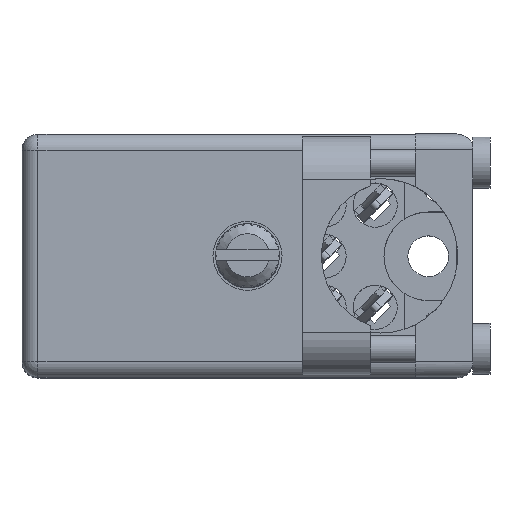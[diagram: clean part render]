
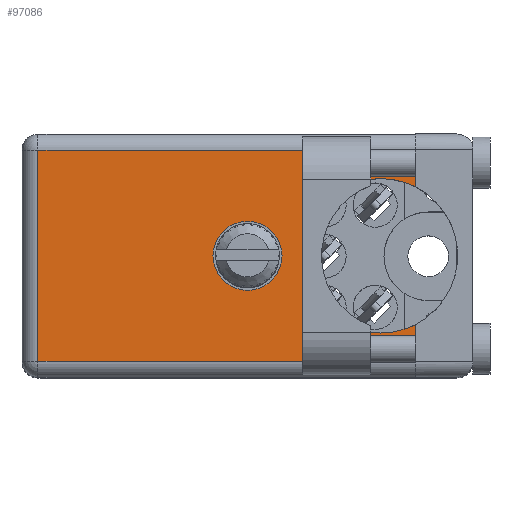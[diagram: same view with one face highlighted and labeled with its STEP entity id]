
A CAD part, top view. The second image highlights one B-rep face of the part: STEP entity #97086.
In plain terms, the highlighted face is planar.
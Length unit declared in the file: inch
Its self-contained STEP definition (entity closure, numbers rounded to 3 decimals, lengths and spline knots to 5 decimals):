
#646 = EDGE_CURVE ( 'NONE', #20752, #139106, #7418, .T. ) ;
#1485 = CARTESIAN_POINT ( 'NONE',  ( 0.6625, 0.906, -0.256 ) ) ;
#4443 = DIRECTION ( 'NONE',  ( 1., 0., 0. ) ) ;
#6586 = EDGE_CURVE ( 'NONE', #76998, #175186, #181791, .T. ) ;
#7418 = CIRCLE ( 'NONE', #58243, 0.227 ) ;
#10437 = CARTESIAN_POINT ( 'NONE',  ( 1.155, 0.906, 0. ) ) ;
#11727 = AXIS2_PLACEMENT_3D ( 'NONE', #88166, #17002, #131221 ) ;
#14114 = CARTESIAN_POINT ( 'NONE',  ( 1.155, 0.906, -0.047 ) ) ;
#14472 = FACE_OUTER_BOUND ( 'NONE', #15183, .T. ) ;
#15183 = EDGE_LOOP ( 'NONE', ( #36356, #139949, #70295, #163960, #52545, #22296, #155546, #24495 ) ) ;
#16550 = CARTESIAN_POINT ( 'NONE',  ( 1.053, 0.906, -0.1305 ) ) ;
#17002 = DIRECTION ( 'NONE',  ( 0., 1., 0. ) ) ;
#20700 = DIRECTION ( 'NONE',  ( 0., 0., 1. ) ) ;
#20752 = VERTEX_POINT ( 'NONE', #16550 ) ;
#22296 = ORIENTED_EDGE ( 'NONE', *, *, #646, .F. ) ;
#24495 = ORIENTED_EDGE ( 'NONE', *, *, #178279, .F. ) ;
#24763 = CIRCLE ( 'NONE', #78447, 0.227 ) ;
#27270 = LINE ( 'NONE', #14114, #47013 ) ;
#29269 = DIRECTION ( 'NONE',  ( 0., 1., 0. ) ) ;
#30152 = CARTESIAN_POINT ( 'NONE',  ( 1.155, 0.906, -0.047 ) ) ;
#33833 = DIRECTION ( 'NONE',  ( 0., 1., 0. ) ) ;
#36356 = ORIENTED_EDGE ( 'NONE', *, *, #183359, .F. ) ;
#37097 = CARTESIAN_POINT ( 'NONE',  ( 0.047, 0.906, -0.668 ) ) ;
#41361 = CARTESIAN_POINT ( 'NONE',  ( 1.053, 0.906, -0.3575 ) ) ;
#44445 = DIRECTION ( 'NONE',  ( 0., 1., 0. ) ) ;
#47013 = VECTOR ( 'NONE', #4443, 39.37008 ) ;
#47773 = VECTOR ( 'NONE', #182708, 39.37008 ) ;
#49642 = CARTESIAN_POINT ( 'NONE',  ( 1.053, 0.906, -0.3575 ) ) ;
#50746 = EDGE_CURVE ( 'NONE', #139106, #70561, #105013, .T. ) ;
#52545 = ORIENTED_EDGE ( 'NONE', *, *, #50746, .F. ) ;
#56371 = CARTESIAN_POINT ( 'NONE',  ( 1.155, 0.906, -0.56029 ) ) ;
#58243 = AXIS2_PLACEMENT_3D ( 'NONE', #49642, #178923, #106756 ) ;
#59424 = VERTEX_POINT ( 'NONE', #1485 ) ;
#65702 = DIRECTION ( 'NONE',  ( 0., 0., 1. ) ) ;
#70295 = ORIENTED_EDGE ( 'NONE', *, *, #6586, .T. ) ;
#70561 = VERTEX_POINT ( 'NONE', #30152 ) ;
#74352 = PLANE ( 'NONE',  #159305 ) ;
#75418 = CARTESIAN_POINT ( 'NONE',  ( 0.047, 0.906, -0.047 ) ) ;
#76998 = VERTEX_POINT ( 'NONE', #37097 ) ;
#77812 = CARTESIAN_POINT ( 'NONE',  ( 0.6625, 0.906, -0.3575 ) ) ;
#78376 = EDGE_CURVE ( 'NONE', #175186, #70561, #27270, .T. ) ;
#78447 = AXIS2_PLACEMENT_3D ( 'NONE', #101325, #29269, #103158 ) ;
#85336 = DIRECTION ( 'NONE',  ( 0., 1., 0. ) ) ;
#87816 = ORIENTED_EDGE ( 'NONE', *, *, #140770, .F. ) ;
#88141 = CIRCLE ( 'NONE', #163008, 0.1015 ) ;
#88166 = CARTESIAN_POINT ( 'NONE',  ( 0.6625, 0.906, -0.3575 ) ) ;
#97086 = ADVANCED_FACE ( 'NONE', ( #14472, #114687 ), #74352, .T. ) ;
#101325 = CARTESIAN_POINT ( 'NONE',  ( 1.053, 0.906, -0.3575 ) ) ;
#102247 = ORIENTED_EDGE ( 'NONE', *, *, #109840, .F. ) ;
#103146 = EDGE_LOOP ( 'NONE', ( #87816, #102247 ) ) ;
#103158 = DIRECTION ( 'NONE',  ( 0., 0., 1. ) ) ;
#105013 = LINE ( 'NONE', #175330, #146068 ) ;
#106756 = DIRECTION ( 'NONE',  ( 0., 0., 1. ) ) ;
#109840 = EDGE_CURVE ( 'NONE', #144207, #59424, #88141, .T. ) ;
#114687 = FACE_BOUND ( 'NONE', #103146, .T. ) ;
#115420 = EDGE_CURVE ( 'NONE', #122422, #76998, #164955, .T. ) ;
#116433 = AXIS2_PLACEMENT_3D ( 'NONE', #41361, #85336, #139667 ) ;
#119280 = VERTEX_POINT ( 'NONE', #56371 ) ;
#122422 = VERTEX_POINT ( 'NONE', #173773 ) ;
#125509 = CARTESIAN_POINT ( 'NONE',  ( 0.047, 0.906, -0.715 ) ) ;
#126523 = LINE ( 'NONE', #10437, #159487 ) ;
#128112 = CARTESIAN_POINT ( 'NONE',  ( 1.053, 0.906, -0.5845 ) ) ;
#129645 = DIRECTION ( 'NONE',  ( 0., 0., 1. ) ) ;
#131221 = DIRECTION ( 'NONE',  ( 0., 0., 1. ) ) ;
#132829 = EDGE_CURVE ( 'NONE', #179733, #20752, #140189, .T. ) ;
#132940 = CARTESIAN_POINT ( 'NONE',  ( 0.6625, 0.906, -0.459 ) ) ;
#134314 = CIRCLE ( 'NONE', #11727, 0.1015 ) ;
#139106 = VERTEX_POINT ( 'NONE', #155406 ) ;
#139667 = DIRECTION ( 'NONE',  ( 0., 0., 1. ) ) ;
#139949 = ORIENTED_EDGE ( 'NONE', *, *, #115420, .T. ) ;
#140189 = CIRCLE ( 'NONE', #116433, 0.227 ) ;
#140770 = EDGE_CURVE ( 'NONE', #59424, #144207, #134314, .T. ) ;
#144207 = VERTEX_POINT ( 'NONE', #132940 ) ;
#146068 = VECTOR ( 'NONE', #146231, 39.37008 ) ;
#146231 = DIRECTION ( 'NONE',  ( 0., 0., 1. ) ) ;
#149011 = DIRECTION ( 'NONE',  ( -1., 0., 0. ) ) ;
#155406 = CARTESIAN_POINT ( 'NONE',  ( 1.155, 0.906, -0.15471 ) ) ;
#155546 = ORIENTED_EDGE ( 'NONE', *, *, #132829, .F. ) ;
#158686 = CARTESIAN_POINT ( 'NONE',  ( 0., 0.906, -0.715 ) ) ;
#159305 = AXIS2_PLACEMENT_3D ( 'NONE', #158686, #44445, #129645 ) ;
#159487 = VECTOR ( 'NONE', #65702, 39.37008 ) ;
#163008 = AXIS2_PLACEMENT_3D ( 'NONE', #77812, #33833, #20700 ) ;
#163276 = VECTOR ( 'NONE', #149011, 39.37008 ) ;
#163960 = ORIENTED_EDGE ( 'NONE', *, *, #78376, .T. ) ;
#164955 = LINE ( 'NONE', #176290, #163276 ) ;
#173773 = CARTESIAN_POINT ( 'NONE',  ( 1.155, 0.906, -0.668 ) ) ;
#175186 = VERTEX_POINT ( 'NONE', #75418 ) ;
#175330 = CARTESIAN_POINT ( 'NONE',  ( 1.155, 0.906, 0. ) ) ;
#176290 = CARTESIAN_POINT ( 'NONE',  ( 0., 0.906, -0.668 ) ) ;
#178279 = EDGE_CURVE ( 'NONE', #119280, #179733, #24763, .T. ) ;
#178923 = DIRECTION ( 'NONE',  ( 0., 1., 0. ) ) ;
#179733 = VERTEX_POINT ( 'NONE', #128112 ) ;
#181791 = LINE ( 'NONE', #125509, #47773 ) ;
#182708 = DIRECTION ( 'NONE',  ( 0., 0., 1. ) ) ;
#183359 = EDGE_CURVE ( 'NONE', #122422, #119280, #126523, .T. ) ;
